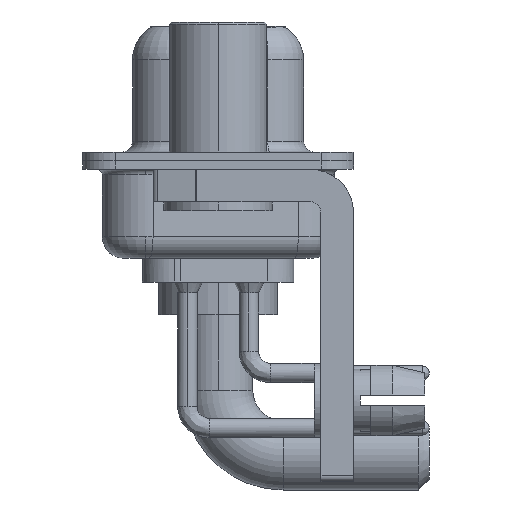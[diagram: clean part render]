
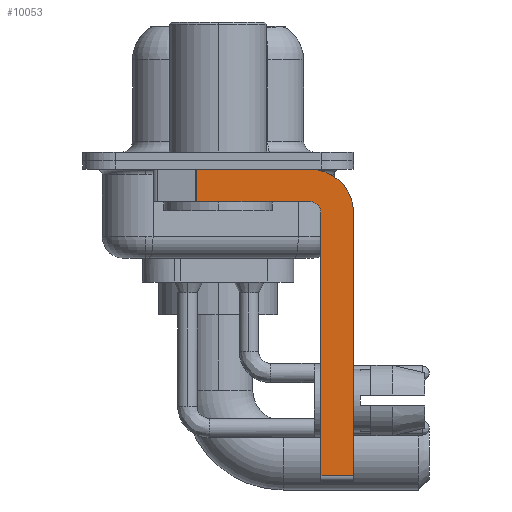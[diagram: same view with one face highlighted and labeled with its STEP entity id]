
A CAD part, left-side view. The second image highlights one B-rep face of the part: STEP entity #10053.
In plain terms, the highlighted planar face has unit normal (-1, 0, 0).
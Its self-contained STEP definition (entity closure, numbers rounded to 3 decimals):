
#477 = ORIENTED_EDGE ( 'NONE', *, *, #17068, .F. ) ;
#577 = EDGE_CURVE ( 'NONE', #9390, #3617, #19614, .T. ) ;
#1201 = CARTESIAN_POINT ( 'NONE',  ( -2.9, -6.25, -2.4 ) ) ;
#1496 = DIRECTION ( 'NONE',  ( 0., 0., -1. ) ) ;
#2151 = EDGE_CURVE ( 'NONE', #8224, #19062, #10042, .T. ) ;
#2806 = CARTESIAN_POINT ( 'NONE',  ( -2.9, -6.25, -2.4 ) ) ;
#3223 = LINE ( 'NONE', #1201, #4092 ) ;
#3617 = VERTEX_POINT ( 'NONE', #2806 ) ;
#3899 = AXIS2_PLACEMENT_3D ( 'NONE', #21969, #24263, #1496 ) ;
#4092 = VECTOR ( 'NONE', #23837, 1000. ) ;
#4162 = ORIENTED_EDGE ( 'NONE', *, *, #25248, .F. ) ;
#4226 = DIRECTION ( 'NONE',  ( 0., 0., 1. ) ) ;
#4596 = EDGE_CURVE ( 'NONE', #8670, #24559, #26722, .T. ) ;
#4671 = CARTESIAN_POINT ( 'NONE',  ( -2.9, -6.25, -14.55 ) ) ;
#4694 = CARTESIAN_POINT ( 'NONE',  ( -2.9, -4.75, -14.55 ) ) ;
#4760 = LINE ( 'NONE', #13035, #19864 ) ;
#5389 = ORIENTED_EDGE ( 'NONE', *, *, #20160, .F. ) ;
#5681 = PLANE ( 'NONE',  #3899 ) ;
#5831 = CARTESIAN_POINT ( 'NONE',  ( -2.9, 0.978, -1.9 ) ) ;
#7617 = CARTESIAN_POINT ( 'NONE',  ( -2.9, -4.25, -2.4 ) ) ;
#8224 = VERTEX_POINT ( 'NONE', #17779 ) ;
#8609 = ORIENTED_EDGE ( 'NONE', *, *, #2151, .T. ) ;
#8623 = EDGE_CURVE ( 'NONE', #9086, #8670, #4760, .T. ) ;
#8670 = VERTEX_POINT ( 'NONE', #23725 ) ;
#8850 = EDGE_CURVE ( 'NONE', #9086, #9488, #9760, .T. ) ;
#8883 = LINE ( 'NONE', #10656, #26606 ) ;
#9086 = VERTEX_POINT ( 'NONE', #4694 ) ;
#9390 = VERTEX_POINT ( 'NONE', #26780 ) ;
#9488 = VERTEX_POINT ( 'NONE', #4671 ) ;
#9760 = LINE ( 'NONE', #18023, #23339 ) ;
#9777 = DIRECTION ( 'NONE',  ( 0., 0., -1. ) ) ;
#10042 = LINE ( 'NONE', #5831, #13209 ) ;
#10053 = ADVANCED_FACE ( 'NONE', ( #19522 ), #5681, .F. ) ;
#10129 = ORIENTED_EDGE ( 'NONE', *, *, #8850, .T. ) ;
#10271 = AXIS2_PLACEMENT_3D ( 'NONE', #15071, #25234, #4226 ) ;
#10495 = ORIENTED_EDGE ( 'NONE', *, *, #577, .F. ) ;
#10656 = CARTESIAN_POINT ( 'NONE',  ( -2.9, 3., -0.4 ) ) ;
#11429 = ORIENTED_EDGE ( 'NONE', *, *, #4596, .F. ) ;
#11674 = DIRECTION ( 'NONE',  ( 1., 0., 0. ) ) ;
#12222 = DIRECTION ( 'NONE',  ( 0., 1., 0. ) ) ;
#12916 = AXIS2_PLACEMENT_3D ( 'NONE', #7617, #11674, #9777 ) ;
#13035 = CARTESIAN_POINT ( 'NONE',  ( -2.9, -4.75, -14.8 ) ) ;
#13209 = VECTOR ( 'NONE', #22522, 1000. ) ;
#13932 = VECTOR ( 'NONE', #12222, 1000. ) ;
#15071 = CARTESIAN_POINT ( 'NONE',  ( -2.9, -4.25, -2.4 ) ) ;
#17068 = EDGE_CURVE ( 'NONE', #24559, #19062, #24274, .T. ) ;
#17779 = CARTESIAN_POINT ( 'NONE',  ( -2.9, 0.978, -0.4 ) ) ;
#18023 = CARTESIAN_POINT ( 'NONE',  ( -2.9, -4.25, -14.55 ) ) ;
#18968 = CARTESIAN_POINT ( 'NONE',  ( -2.9, 0.978, -1.9 ) ) ;
#19062 = VERTEX_POINT ( 'NONE', #18968 ) ;
#19522 = FACE_OUTER_BOUND ( 'NONE', #20764, .T. ) ;
#19614 = CIRCLE ( 'NONE', #12916, 2. ) ;
#19864 = VECTOR ( 'NONE', #21300, 1000. ) ;
#19989 = CARTESIAN_POINT ( 'NONE',  ( -2.9, -4.25, -1.9 ) ) ;
#20160 = EDGE_CURVE ( 'NONE', #8224, #9390, #8883, .T. ) ;
#20764 = EDGE_LOOP ( 'NONE', ( #5389, #8609, #477, #11429, #24935, #10129, #4162, #10495 ) ) ;
#21091 = DIRECTION ( 'NONE',  ( 0., -1., 0. ) ) ;
#21300 = DIRECTION ( 'NONE',  ( 0., 0., 1. ) ) ;
#21969 = CARTESIAN_POINT ( 'NONE',  ( -2.9, -4.25, -2.4 ) ) ;
#22522 = DIRECTION ( 'NONE',  ( 0., 0., -1. ) ) ;
#23339 = VECTOR ( 'NONE', #26567, 1000. ) ;
#23725 = CARTESIAN_POINT ( 'NONE',  ( -2.9, -4.75, -2.4 ) ) ;
#23837 = DIRECTION ( 'NONE',  ( 0., 0., -1. ) ) ;
#24263 = DIRECTION ( 'NONE',  ( 1., 0., 0. ) ) ;
#24274 = LINE ( 'NONE', #26322, #13932 ) ;
#24559 = VERTEX_POINT ( 'NONE', #19989 ) ;
#24935 = ORIENTED_EDGE ( 'NONE', *, *, #8623, .F. ) ;
#25234 = DIRECTION ( 'NONE',  ( -1., 0., 0. ) ) ;
#25248 = EDGE_CURVE ( 'NONE', #3617, #9488, #3223, .T. ) ;
#26322 = CARTESIAN_POINT ( 'NONE',  ( -2.9, -4.25, -1.9 ) ) ;
#26567 = DIRECTION ( 'NONE',  ( 0., -1., 0. ) ) ;
#26606 = VECTOR ( 'NONE', #21091, 1000. ) ;
#26722 = CIRCLE ( 'NONE', #10271, 0.5 ) ;
#26780 = CARTESIAN_POINT ( 'NONE',  ( -2.9, -4.25, -0.4 ) ) ;
